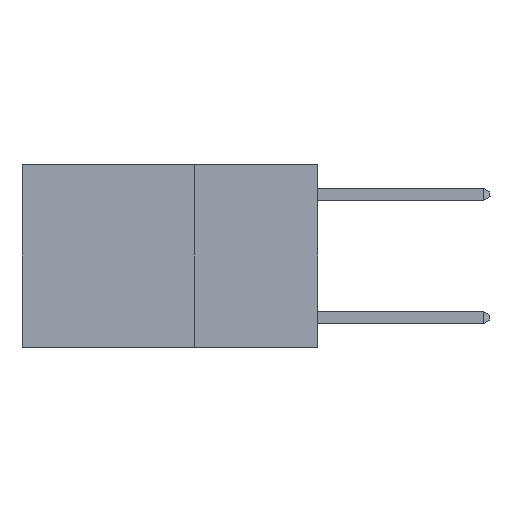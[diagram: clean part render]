
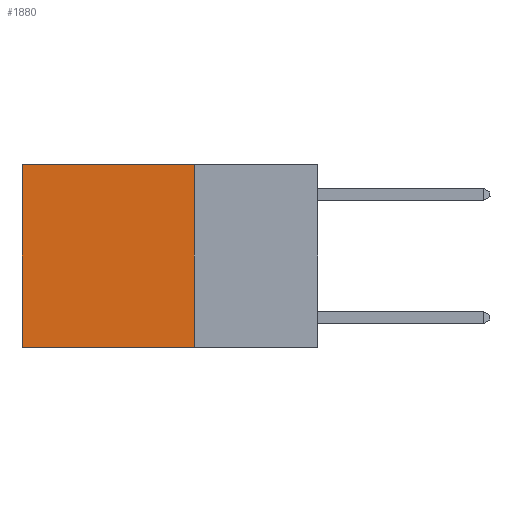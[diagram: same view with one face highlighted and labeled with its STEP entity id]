
A CAD part, left-side view. The second image highlights one B-rep face of the part: STEP entity #1880.
In plain terms, the highlighted planar face has unit normal (-1, 0, 0).
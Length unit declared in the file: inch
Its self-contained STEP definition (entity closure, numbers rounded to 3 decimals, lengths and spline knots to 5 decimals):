
#638 = LINE ( 'NONE', #6337, #9618 ) ;
#837 = LINE ( 'NONE', #2849, #9550 ) ;
#1430 = ORIENTED_EDGE ( 'NONE', *, *, #6210, .T. ) ;
#1474 = DIRECTION ( 'NONE',  ( 0., 1., 0. ) ) ;
#1504 = CARTESIAN_POINT ( 'NONE',  ( 0.2625, 0.6, 0. ) ) ;
#1703 = DIRECTION ( 'NONE',  ( 0., 0., -1. ) ) ;
#1876 = CARTESIAN_POINT ( 'NONE',  ( 0.2625, 0.6, 0. ) ) ;
#1880 = ADVANCED_FACE ( 'NONE', ( #7181 ), #2582, .F. ) ;
#2361 = LINE ( 'NONE', #11999, #9334 ) ;
#2582 = PLANE ( 'NONE',  #8152 ) ;
#2747 = ORIENTED_EDGE ( 'NONE', *, *, #11541, .F. ) ;
#2849 = CARTESIAN_POINT ( 'NONE',  ( 0.2625, 0.25, -0.37 ) ) ;
#3438 = VERTEX_POINT ( 'NONE', #7043 ) ;
#3538 = VERTEX_POINT ( 'NONE', #11180 ) ;
#4601 = DIRECTION ( 'NONE',  ( 1., 0., 0. ) ) ;
#5289 = VERTEX_POINT ( 'NONE', #8872 ) ;
#5487 = VECTOR ( 'NONE', #10487, 39.37008 ) ;
#6210 = EDGE_CURVE ( 'NONE', #5289, #9268, #2361, .T. ) ;
#6337 = CARTESIAN_POINT ( 'NONE',  ( 0.2625, 0.25, 0. ) ) ;
#7043 = CARTESIAN_POINT ( 'NONE',  ( 0.2625, 0.6, -0.37 ) ) ;
#7181 = FACE_OUTER_BOUND ( 'NONE', #10288, .T. ) ;
#7543 = LINE ( 'NONE', #1876, #5487 ) ;
#8092 = ORIENTED_EDGE ( 'NONE', *, *, #10762, .T. ) ;
#8152 = AXIS2_PLACEMENT_3D ( 'NONE', #9054, #4601, #1703 ) ;
#8268 = ORIENTED_EDGE ( 'NONE', *, *, #8837, .F. ) ;
#8634 = DIRECTION ( 'NONE',  ( 0., 1., 0. ) ) ;
#8837 = EDGE_CURVE ( 'NONE', #5289, #3538, #638, .T. ) ;
#8872 = CARTESIAN_POINT ( 'NONE',  ( 0.2625, 0.25, 0. ) ) ;
#9054 = CARTESIAN_POINT ( 'NONE',  ( 0.2625, 0.25, 0. ) ) ;
#9181 = DIRECTION ( 'NONE',  ( 0., 0., -1. ) ) ;
#9268 = VERTEX_POINT ( 'NONE', #1504 ) ;
#9334 = VECTOR ( 'NONE', #1474, 39.37008 ) ;
#9550 = VECTOR ( 'NONE', #8634, 39.37008 ) ;
#9618 = VECTOR ( 'NONE', #9181, 39.37008 ) ;
#10288 = EDGE_LOOP ( 'NONE', ( #8092, #2747, #8268, #1430 ) ) ;
#10487 = DIRECTION ( 'NONE',  ( 0., 0., -1. ) ) ;
#10762 = EDGE_CURVE ( 'NONE', #9268, #3438, #7543, .T. ) ;
#11180 = CARTESIAN_POINT ( 'NONE',  ( 0.2625, 0.25, -0.37 ) ) ;
#11541 = EDGE_CURVE ( 'NONE', #3538, #3438, #837, .T. ) ;
#11999 = CARTESIAN_POINT ( 'NONE',  ( 0.2625, 0.25, 0. ) ) ;
